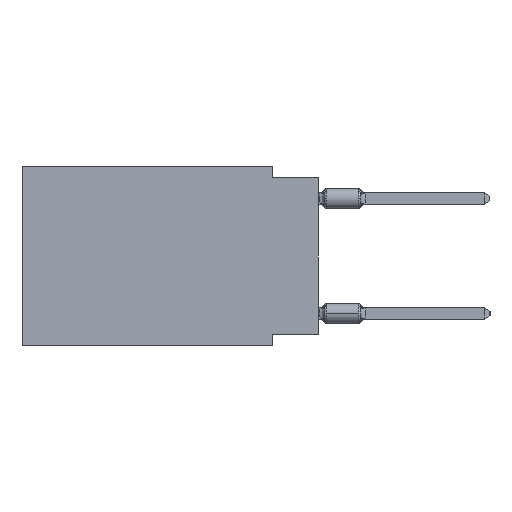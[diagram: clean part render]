
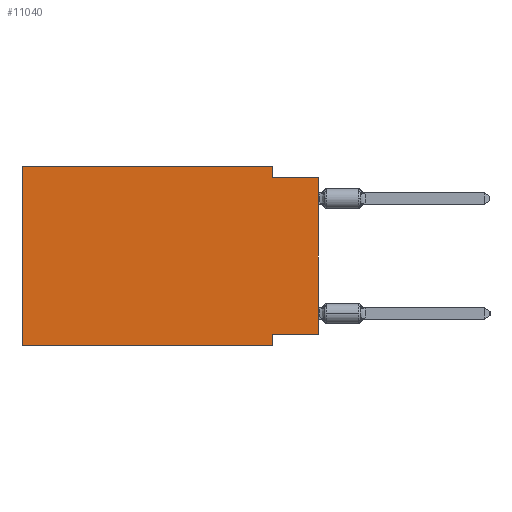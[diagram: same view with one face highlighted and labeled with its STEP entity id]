
A CAD part, left-side view. The second image highlights one B-rep face of the part: STEP entity #11040.
In plain terms, the highlighted planar face has unit normal (-1, 0, 0).
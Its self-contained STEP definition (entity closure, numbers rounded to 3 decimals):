
#639 = DIRECTION ( 'NONE',  ( 0., 0., 1. ) ) ;
#648 = VERTEX_POINT ( 'NONE', #33619 ) ;
#1295 = VERTEX_POINT ( 'NONE', #13563 ) ;
#1850 = ORIENTED_EDGE ( 'NONE', *, *, #26766, .F. ) ;
#3047 = DIRECTION ( 'NONE',  ( 0., 0., -1. ) ) ;
#4273 = CARTESIAN_POINT ( 'NONE',  ( 0., 16.383, 0. ) ) ;
#4313 = VECTOR ( 'NONE', #30745, 1000. ) ;
#4477 = CARTESIAN_POINT ( 'NONE',  ( 0., 0., -0.635 ) ) ;
#4672 = VERTEX_POINT ( 'NONE', #23325 ) ;
#5730 = CARTESIAN_POINT ( 'NONE',  ( 0., 16.383, -9.906 ) ) ;
#5904 = CARTESIAN_POINT ( 'NONE',  ( 0., 2.54, -9.906 ) ) ;
#7063 = VECTOR ( 'NONE', #3047, 1000. ) ;
#7294 = EDGE_CURVE ( 'NONE', #4672, #1295, #11976, .T. ) ;
#7736 = CARTESIAN_POINT ( 'NONE',  ( 0., 16.383, -9.906 ) ) ;
#7970 = EDGE_CURVE ( 'NONE', #12547, #648, #14973, .T. ) ;
#8868 = DIRECTION ( 'NONE',  ( 0., -1., 0. ) ) ;
#9256 = CARTESIAN_POINT ( 'NONE',  ( 0., 2.54, -9.271 ) ) ;
#10860 = LINE ( 'NONE', #22264, #23654 ) ;
#11040 = ADVANCED_FACE ( 'NONE', ( #13303 ), #17438, .F. ) ;
#11780 = LINE ( 'NONE', #4477, #33545 ) ;
#11976 = LINE ( 'NONE', #38192, #27521 ) ;
#12547 = VERTEX_POINT ( 'NONE', #5730 ) ;
#13303 = FACE_OUTER_BOUND ( 'NONE', #20683, .T. ) ;
#13563 = CARTESIAN_POINT ( 'NONE',  ( 0., 2.54, -0.635 ) ) ;
#13656 = LINE ( 'NONE', #35258, #23548 ) ;
#14063 = EDGE_CURVE ( 'NONE', #1295, #14238, #11780, .T. ) ;
#14238 = VERTEX_POINT ( 'NONE', #16625 ) ;
#14276 = CARTESIAN_POINT ( 'NONE',  ( 0., 16.383, 0. ) ) ;
#14973 = LINE ( 'NONE', #4273, #15887 ) ;
#15887 = VECTOR ( 'NONE', #639, 1000. ) ;
#16559 = DIRECTION ( 'NONE',  ( 0., -1., 0. ) ) ;
#16625 = CARTESIAN_POINT ( 'NONE',  ( 0., 0., -0.635 ) ) ;
#16713 = AXIS2_PLACEMENT_3D ( 'NONE', #14276, #29089, #21333 ) ;
#17071 = EDGE_CURVE ( 'NONE', #18281, #14238, #10860, .T. ) ;
#17438 = PLANE ( 'NONE',  #16713 ) ;
#18281 = VERTEX_POINT ( 'NONE', #30259 ) ;
#20683 = EDGE_LOOP ( 'NONE', ( #31018, #22192, #47053, #1850, #33138, #46698, #43115, #22717 ) ) ;
#21333 = DIRECTION ( 'NONE',  ( 0., 0., -1. ) ) ;
#22087 = LINE ( 'NONE', #7736, #37115 ) ;
#22192 = ORIENTED_EDGE ( 'NONE', *, *, #14063, .F. ) ;
#22264 = CARTESIAN_POINT ( 'NONE',  ( 0., 0., 0. ) ) ;
#22717 = ORIENTED_EDGE ( 'NONE', *, *, #39223, .F. ) ;
#23325 = CARTESIAN_POINT ( 'NONE',  ( 0., 2.54, 0. ) ) ;
#23548 = VECTOR ( 'NONE', #16559, 1000. ) ;
#23654 = VECTOR ( 'NONE', #37059, 1000. ) ;
#23999 = EDGE_CURVE ( 'NONE', #12547, #39640, #22087, .T. ) ;
#26766 = EDGE_CURVE ( 'NONE', #648, #4672, #13656, .T. ) ;
#27521 = VECTOR ( 'NONE', #30907, 1000. ) ;
#29089 = DIRECTION ( 'NONE',  ( 1., 0., 0. ) ) ;
#30259 = CARTESIAN_POINT ( 'NONE',  ( 0., 0., -9.271 ) ) ;
#30304 = DIRECTION ( 'NONE',  ( 0., -1., 0. ) ) ;
#30745 = DIRECTION ( 'NONE',  ( 0., 1., 0. ) ) ;
#30907 = DIRECTION ( 'NONE',  ( 0., 0., -1. ) ) ;
#31018 = ORIENTED_EDGE ( 'NONE', *, *, #17071, .T. ) ;
#31231 = CARTESIAN_POINT ( 'NONE',  ( 0., 0., -9.271 ) ) ;
#32449 = CARTESIAN_POINT ( 'NONE',  ( 0., 2.54, -9.906 ) ) ;
#32682 = LINE ( 'NONE', #32449, #7063 ) ;
#33138 = ORIENTED_EDGE ( 'NONE', *, *, #7970, .F. ) ;
#33545 = VECTOR ( 'NONE', #8868, 1000. ) ;
#33619 = CARTESIAN_POINT ( 'NONE',  ( 0., 16.383, 0. ) ) ;
#35258 = CARTESIAN_POINT ( 'NONE',  ( 0., 16.383, 0. ) ) ;
#37059 = DIRECTION ( 'NONE',  ( 0., 0., 1. ) ) ;
#37115 = VECTOR ( 'NONE', #30304, 1000. ) ;
#38012 = LINE ( 'NONE', #31231, #4313 ) ;
#38192 = CARTESIAN_POINT ( 'NONE',  ( 0., 2.54, 0. ) ) ;
#39223 = EDGE_CURVE ( 'NONE', #18281, #45385, #38012, .T. ) ;
#39640 = VERTEX_POINT ( 'NONE', #5904 ) ;
#43115 = ORIENTED_EDGE ( 'NONE', *, *, #47681, .F. ) ;
#45385 = VERTEX_POINT ( 'NONE', #9256 ) ;
#46698 = ORIENTED_EDGE ( 'NONE', *, *, #23999, .T. ) ;
#47053 = ORIENTED_EDGE ( 'NONE', *, *, #7294, .F. ) ;
#47681 = EDGE_CURVE ( 'NONE', #45385, #39640, #32682, .T. ) ;
